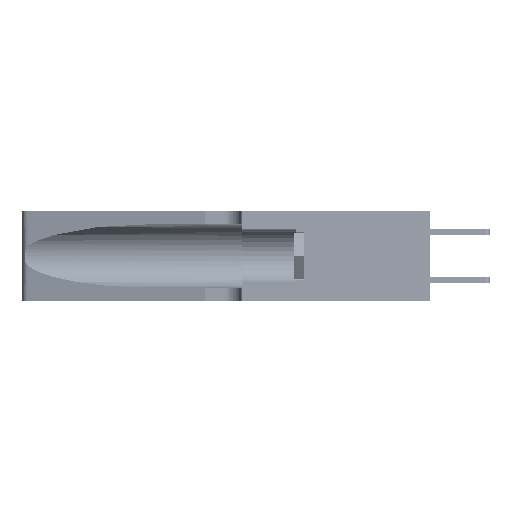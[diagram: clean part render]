
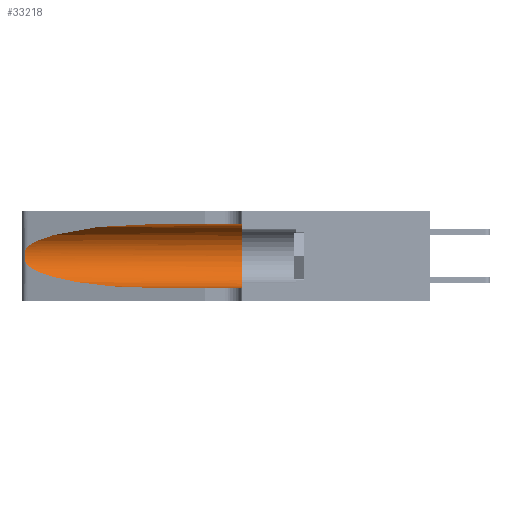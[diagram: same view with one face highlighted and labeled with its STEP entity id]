
A CAD part, left-side view. The second image highlights one B-rep face of the part: STEP entity #33218.
In plain terms, the highlighted cylindrical face has radius 3.308 mm (diameter 6.617 mm), a partial arc.
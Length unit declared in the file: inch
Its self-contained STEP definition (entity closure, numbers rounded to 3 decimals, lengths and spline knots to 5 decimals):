
#1064 = AXIS2_PLACEMENT_3D ( 'NONE', #42451, #15536, #23543 ) ;
#2436 = LINE ( 'NONE', #34963, #30594 ) ;
#3277 = CARTESIAN_POINT ( 'NONE',  ( 0.25555, 1.22993, 0.14849 ) ) ;
#3603 = CARTESIAN_POINT ( 'NONE',  ( 0.26075, 1.23896, 0.19203 ) ) ;
#3759 = CARTESIAN_POINT ( 'NONE',  ( 0.26018, 1.23835, 0.19895 ) ) ;
#3861 = VERTEX_POINT ( 'NONE', #12817 ) ;
#5019 = CARTESIAN_POINT ( 'NONE',  ( 0.25487, 1.22718, 0.14631 ) ) ;
#5046 = CARTESIAN_POINT ( 'NONE',  ( 0.1305, 0.35, 0.31525 ) ) ;
#5885 = CARTESIAN_POINT ( 'NONE',  ( 0.1305, 0.72297, 0.31525 ) ) ;
#6867 = ORIENTED_EDGE ( 'NONE', *, *, #26940, .T. ) ;
#7133 = CARTESIAN_POINT ( 'NONE',  ( 0.25555, 1.22994, 0.2215 ) ) ;
#7795 = CARTESIAN_POINT ( 'NONE',  ( 0.26017, 1.23833, 0.17102 ) ) ;
#8386 = CARTESIAN_POINT ( 'NONE',  ( 0.18966, 0.96281, 0.05475 ) ) ;
#9504 = EDGE_LOOP ( 'NONE', ( #6867, #37427, #48164, #12864, #27252, #34378 ) ) ;
#10117 = CARTESIAN_POINT ( 'NONE',  ( 0.1305, 0.72297, 0.05475 ) ) ;
#10177 = CARTESIAN_POINT ( 'NONE',  ( 0.1305, 0.72297, 0.31525 ) ) ;
#11434 = EDGE_CURVE ( 'NONE', #28306, #3861, #44489, .T. ) ;
#11662 = CARTESIAN_POINT ( 'NONE',  ( 0.25639, 1.23186, 0.15144 ) ) ;
#12521 = EDGE_CURVE ( 'NONE', #45212, #3861, #2436, .T. ) ;
#12817 = CARTESIAN_POINT ( 'NONE',  ( 0.1305, 0.35, 0.05475 ) ) ;
#12864 = ORIENTED_EDGE ( 'NONE', *, *, #12521, .T. ) ;
#13627 = CARTESIAN_POINT ( 'NONE',  ( 0.2373, 1.15595, 0.28018 ) ) ;
#14652 = DIRECTION ( 'NONE',  ( 0., 0., -1. ) ) ;
#15010 = CARTESIAN_POINT ( 'NONE',  ( 0.25854, 1.2359, 0.20912 ) ) ;
#15536 = DIRECTION ( 'NONE',  ( 0., 1., 0. ) ) ;
#16254 = CARTESIAN_POINT ( 'NONE',  ( 0.25487, 1.22718, 0.14631 ) ) ;
#16728 = EDGE_CURVE ( 'NONE', #30630, #34410, #26160, .T. ) ;
#18046 = AXIS2_PLACEMENT_3D ( 'NONE', #22339, #37560, #14652 ) ;
#19766 = DIRECTION ( 'NONE',  ( 0., -1., 0. ) ) ;
#22339 = CARTESIAN_POINT ( 'NONE',  ( 0.1305, 1.61858, 0.185 ) ) ;
#22706 = CARTESIAN_POINT ( 'NONE',  ( 0.25856, 1.23593, 0.16098 ) ) ;
#23543 = DIRECTION ( 'NONE',  ( 0., 0., 1. ) ) ;
#25274 = LINE ( 'NONE', #34501, #49184 ) ;
#26160 = B_SPLINE_CURVE_WITH_KNOTS ( 'NONE', 3,
 ( #26214, #7133, #26530, #45442, #15010, #3759, #3603, #30709, #7795, #22706, #34559, #11662, #3277, #41768 ),
 .UNSPECIFIED., .F., .F.,
 ( 4, 2, 2, 2, 2, 2, 4 ),
 ( 0., 0.00027, 0.00053, 0.00107, 0.0016, 0.00187, 0.00214 ),
 .UNSPECIFIED. ) ;
#26214 = CARTESIAN_POINT ( 'NONE',  ( 0.25487, 1.22718, 0.22369 ) ) ;
#26530 = CARTESIAN_POINT ( 'NONE',  ( 0.25639, 1.23184, 0.21858 ) ) ;
#26940 = EDGE_CURVE ( 'NONE', #49305, #30630, #44850, .T. ) ;
#27119 = FACE_OUTER_BOUND ( 'NONE', #9504, .T. ) ;
#27252 = ORIENTED_EDGE ( 'NONE', *, *, #11434, .F. ) ;
#28306 = VERTEX_POINT ( 'NONE', #5046 ) ;
#30594 = VECTOR ( 'NONE', #19766, 39.37008 ) ;
#30630 = VERTEX_POINT ( 'NONE', #45266 ) ;
#30709 = CARTESIAN_POINT ( 'NONE',  ( 0.26075, 1.23896, 0.178 ) ) ;
#31466 = CARTESIAN_POINT ( 'NONE',  ( 0.1305, 0.72297, 0.05475 ) ) ;
#33218 = ADVANCED_FACE ( 'NONE', ( #27119 ), #37314, .F. ) ;
#33684 = CARTESIAN_POINT ( 'NONE',  ( 0.18966, 0.96281, 0.31525 ) ) ;
#34378 = ORIENTED_EDGE ( 'NONE', *, *, #39976, .F. ) ;
#34410 = VERTEX_POINT ( 'NONE', #5019 ) ;
#34501 = CARTESIAN_POINT ( 'NONE',  ( 0.1305, 1.61858, 0.31525 ) ) ;
#34559 = CARTESIAN_POINT ( 'NONE',  ( 0.25789, 1.23486, 0.15765 ) ) ;
#34809 = CARTESIAN_POINT ( 'NONE',  ( 0.2373, 1.15595, 0.08982 ) ) ;
#34963 = CARTESIAN_POINT ( 'NONE',  ( 0.1305, 1.61858, 0.05475 ) ) ;
#37314 = CYLINDRICAL_SURFACE ( 'NONE', #18046, 0.13025 ) ;
#37427 = ORIENTED_EDGE ( 'NONE', *, *, #16728, .T. ) ;
#37560 = DIRECTION ( 'NONE',  ( 0., -1., 0. ) ) ;
#39976 = EDGE_CURVE ( 'NONE', #49305, #28306, #25274, .T. ) ;
#40349 = CARTESIAN_POINT ( 'NONE',  ( 0.25487, 1.22718, 0.22369 ) ) ;
#41768 = CARTESIAN_POINT ( 'NONE',  ( 0.25487, 1.22718, 0.14631 ) ) ;
#42451 = CARTESIAN_POINT ( 'NONE',  ( 0.1305, 0.35, 0.185 ) ) ;
#44489 = CIRCLE ( 'NONE', #1064, 0.13025 ) ;
#44850 =( BOUNDED_CURVE ( )  B_SPLINE_CURVE ( 3, ( #5885, #33684, #13627, #40349 ),
 .UNSPECIFIED., .F., .T. ) 
 B_SPLINE_CURVE_WITH_KNOTS ( ( 4, 4 ),
 ( 1.5708, 2.84003 ),
 .UNSPECIFIED. ) 
 CURVE ( )  GEOMETRIC_REPRESENTATION_ITEM ( )  RATIONAL_B_SPLINE_CURVE ( ( 1., 0.87, 0.87, 1. ) ) 
 REPRESENTATION_ITEM ( '' )  );
#45212 = VERTEX_POINT ( 'NONE', #10117 ) ;
#45266 = CARTESIAN_POINT ( 'NONE',  ( 0.25487, 1.22718, 0.22369 ) ) ;
#45442 = CARTESIAN_POINT ( 'NONE',  ( 0.25787, 1.23484, 0.2124 ) ) ;
#45472 =( BOUNDED_CURVE ( )  B_SPLINE_CURVE ( 3, ( #16254, #34809, #8386, #31466 ),
 .UNSPECIFIED., .F., .T. ) 
 B_SPLINE_CURVE_WITH_KNOTS ( ( 4, 4 ),
 ( 3.44316, 4.71239 ),
 .UNSPECIFIED. ) 
 CURVE ( )  GEOMETRIC_REPRESENTATION_ITEM ( )  RATIONAL_B_SPLINE_CURVE ( ( 1., 0.87, 0.87, 1. ) ) 
 REPRESENTATION_ITEM ( '' )  );
#45874 = DIRECTION ( 'NONE',  ( 0., -1., 0. ) ) ;
#48164 = ORIENTED_EDGE ( 'NONE', *, *, #49094, .T. ) ;
#49094 = EDGE_CURVE ( 'NONE', #34410, #45212, #45472, .T. ) ;
#49184 = VECTOR ( 'NONE', #45874, 39.37008 ) ;
#49305 = VERTEX_POINT ( 'NONE', #10177 ) ;
